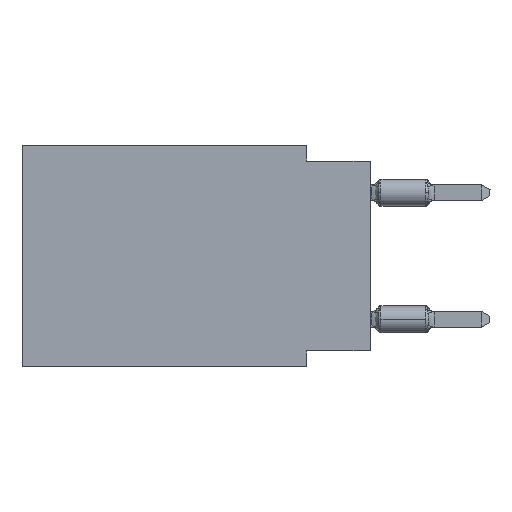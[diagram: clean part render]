
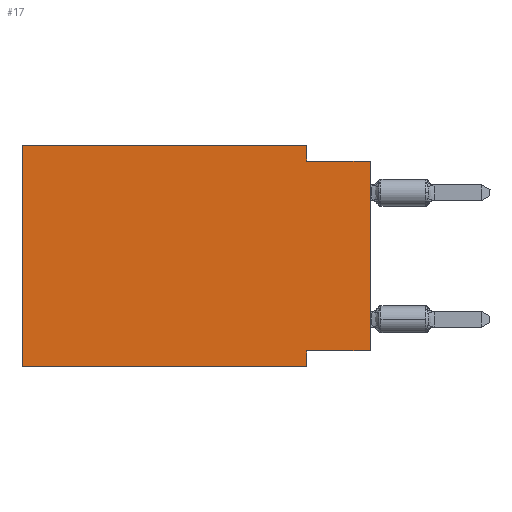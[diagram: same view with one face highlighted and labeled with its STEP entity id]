
A CAD part, left-side view. The second image highlights one B-rep face of the part: STEP entity #17.
In plain terms, the highlighted planar face has unit normal (-1, 0, 0).
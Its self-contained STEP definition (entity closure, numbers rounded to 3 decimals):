
#17 = ADVANCED_FACE ( 'NONE', ( #5435 ), #3781, .F. ) ;
#55 = DIRECTION ( 'NONE',  ( 0., 0., 1. ) ) ;
#292 = DIRECTION ( 'NONE',  ( 0., 0., -1. ) ) ;
#484 = ORIENTED_EDGE ( 'NONE', *, *, #7965, .F. ) ;
#554 = EDGE_CURVE ( 'NONE', #3725, #9813, #9221, .T. ) ;
#694 = EDGE_LOOP ( 'NONE', ( #1234, #21365, #1181, #10866, #484, #20716, #9729, #19009 ) ) ;
#770 = VECTOR ( 'NONE', #2260, 1000. ) ;
#1181 = ORIENTED_EDGE ( 'NONE', *, *, #14098, .F. ) ;
#1230 = EDGE_CURVE ( 'NONE', #2813, #19582, #10282, .T. ) ;
#1234 = ORIENTED_EDGE ( 'NONE', *, *, #20939, .T. ) ;
#1510 = VECTOR ( 'NONE', #55, 1000. ) ;
#1588 = VERTEX_POINT ( 'NONE', #6296 ) ;
#1607 = LINE ( 'NONE', #8323, #14662 ) ;
#1699 = VECTOR ( 'NONE', #292, 1000. ) ;
#1913 = DIRECTION ( 'NONE',  ( 0., 0., -1. ) ) ;
#2260 = DIRECTION ( 'NONE',  ( 0., -1., 0. ) ) ;
#2727 = CARTESIAN_POINT ( 'NONE',  ( 0., 2.54, -8.89 ) ) ;
#2813 = VERTEX_POINT ( 'NONE', #3836 ) ;
#3176 = VECTOR ( 'NONE', #11963, 1000. ) ;
#3606 = LINE ( 'NONE', #12191, #3176 ) ;
#3725 = VERTEX_POINT ( 'NONE', #4103 ) ;
#3781 = PLANE ( 'NONE',  #8916 ) ;
#3816 = CARTESIAN_POINT ( 'NONE',  ( 0., 2.54, 0. ) ) ;
#3836 = CARTESIAN_POINT ( 'NONE',  ( 0., 2.54, -0.635 ) ) ;
#4103 = CARTESIAN_POINT ( 'NONE',  ( 0., 0., -8.255 ) ) ;
#4126 = EDGE_CURVE ( 'NONE', #9813, #4948, #12863, .T. ) ;
#4948 = VERTEX_POINT ( 'NONE', #12589 ) ;
#5435 = FACE_OUTER_BOUND ( 'NONE', #694, .T. ) ;
#5567 = LINE ( 'NONE', #12281, #770 ) ;
#6296 = CARTESIAN_POINT ( 'NONE',  ( 0., 13.97, 0. ) ) ;
#6557 = DIRECTION ( 'NONE',  ( 0., 0., 1. ) ) ;
#6758 = DIRECTION ( 'NONE',  ( 0., -1., 0. ) ) ;
#7965 = EDGE_CURVE ( 'NONE', #18030, #1588, #13302, .T. ) ;
#8107 = EDGE_CURVE ( 'NONE', #18030, #4948, #5567, .T. ) ;
#8323 = CARTESIAN_POINT ( 'NONE',  ( 0., 0., 0. ) ) ;
#8435 = CARTESIAN_POINT ( 'NONE',  ( 0., 13.97, 0. ) ) ;
#8916 = AXIS2_PLACEMENT_3D ( 'NONE', #12147, #17017, #1913 ) ;
#9221 = LINE ( 'NONE', #19373, #14210 ) ;
#9729 = ORIENTED_EDGE ( 'NONE', *, *, #4126, .F. ) ;
#9813 = VERTEX_POINT ( 'NONE', #21181 ) ;
#9885 = CARTESIAN_POINT ( 'NONE',  ( 0., 2.54, 0. ) ) ;
#10237 = CARTESIAN_POINT ( 'NONE',  ( 0., 13.97, -8.89 ) ) ;
#10282 = LINE ( 'NONE', #18666, #14587 ) ;
#10536 = CARTESIAN_POINT ( 'NONE',  ( 0., 0., -0.635 ) ) ;
#10866 = ORIENTED_EDGE ( 'NONE', *, *, #16821, .F. ) ;
#11963 = DIRECTION ( 'NONE',  ( 0., -1., 0. ) ) ;
#12147 = CARTESIAN_POINT ( 'NONE',  ( 0., 13.97, 0. ) ) ;
#12191 = CARTESIAN_POINT ( 'NONE',  ( 0., 13.97, 0. ) ) ;
#12281 = CARTESIAN_POINT ( 'NONE',  ( 0., 13.97, -8.89 ) ) ;
#12589 = CARTESIAN_POINT ( 'NONE',  ( 0., 2.54, -8.89 ) ) ;
#12860 = DIRECTION ( 'NONE',  ( 0., 1., 0. ) ) ;
#12863 = LINE ( 'NONE', #2727, #20839 ) ;
#13302 = LINE ( 'NONE', #8435, #1510 ) ;
#14098 = EDGE_CURVE ( 'NONE', #16721, #2813, #15399, .T. ) ;
#14210 = VECTOR ( 'NONE', #12860, 1000. ) ;
#14587 = VECTOR ( 'NONE', #6758, 1000. ) ;
#14662 = VECTOR ( 'NONE', #6557, 1000. ) ;
#15399 = LINE ( 'NONE', #3816, #1699 ) ;
#16721 = VERTEX_POINT ( 'NONE', #9885 ) ;
#16821 = EDGE_CURVE ( 'NONE', #1588, #16721, #3606, .T. ) ;
#17017 = DIRECTION ( 'NONE',  ( 1., 0., 0. ) ) ;
#18030 = VERTEX_POINT ( 'NONE', #10237 ) ;
#18666 = CARTESIAN_POINT ( 'NONE',  ( 0., 0., -0.635 ) ) ;
#19009 = ORIENTED_EDGE ( 'NONE', *, *, #554, .F. ) ;
#19373 = CARTESIAN_POINT ( 'NONE',  ( 0., 0., -8.255 ) ) ;
#19485 = DIRECTION ( 'NONE',  ( 0., 0., -1. ) ) ;
#19582 = VERTEX_POINT ( 'NONE', #10536 ) ;
#20716 = ORIENTED_EDGE ( 'NONE', *, *, #8107, .T. ) ;
#20839 = VECTOR ( 'NONE', #19485, 1000. ) ;
#20939 = EDGE_CURVE ( 'NONE', #3725, #19582, #1607, .T. ) ;
#21181 = CARTESIAN_POINT ( 'NONE',  ( 0., 2.54, -8.255 ) ) ;
#21365 = ORIENTED_EDGE ( 'NONE', *, *, #1230, .F. ) ;
